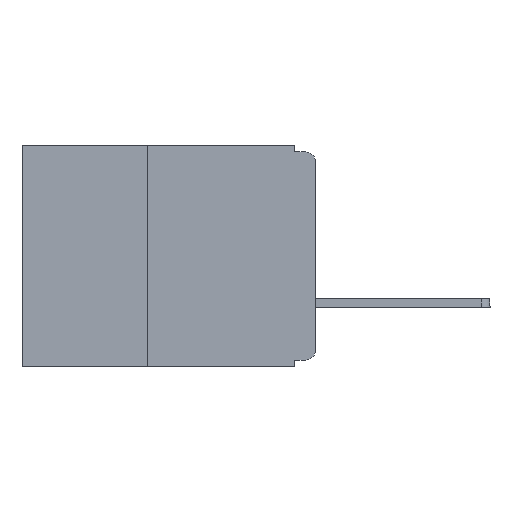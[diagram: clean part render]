
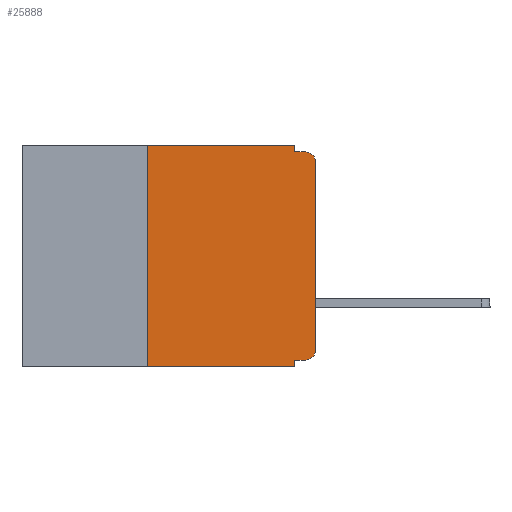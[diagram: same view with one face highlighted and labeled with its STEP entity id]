
A CAD part, left-side view. The second image highlights one B-rep face of the part: STEP entity #25888.
In plain terms, the highlighted planar face has unit normal (-1, 0, 0).
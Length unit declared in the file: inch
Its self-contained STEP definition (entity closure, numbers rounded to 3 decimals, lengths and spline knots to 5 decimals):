
#901 = AXIS2_PLACEMENT_3D ( 'NONE', #1587, #17180, #3846 ) ;
#1143 = CARTESIAN_POINT ( 'NONE',  ( 0., 0.015, -0.01 ) ) ;
#1209 = VECTOR ( 'NONE', #21143, 39.37008 ) ;
#1587 = CARTESIAN_POINT ( 'NONE',  ( 0., 0.015, -0.305 ) ) ;
#1785 = VERTEX_POINT ( 'NONE', #26968 ) ;
#2068 = VECTOR ( 'NONE', #14072, 39.37008 ) ;
#3245 = DIRECTION ( 'NONE',  ( 0., 0., 1. ) ) ;
#3846 = DIRECTION ( 'NONE',  ( 0., 0., -1. ) ) ;
#4267 = ORIENTED_EDGE ( 'NONE', *, *, #18179, .F. ) ;
#4443 = EDGE_CURVE ( 'NONE', #26422, #20674, #8044, .T. ) ;
#4678 = DIRECTION ( 'NONE',  ( 0., -1., 0. ) ) ;
#4700 = AXIS2_PLACEMENT_3D ( 'NONE', #23439, #10240, #25646 ) ;
#4774 = CARTESIAN_POINT ( 'NONE',  ( 0., 0.031, -0.01 ) ) ;
#4798 = CARTESIAN_POINT ( 'NONE',  ( 0., 0., -0.305 ) ) ;
#5119 = CARTESIAN_POINT ( 'NONE',  ( 0., 0.25, -0.33 ) ) ;
#5506 = EDGE_CURVE ( 'NONE', #12307, #23863, #15617, .T. ) ;
#5645 = CARTESIAN_POINT ( 'NONE',  ( 0., 0., -0.32 ) ) ;
#5861 = ORIENTED_EDGE ( 'NONE', *, *, #8614, .T. ) ;
#6112 = CARTESIAN_POINT ( 'NONE',  ( 0., 0.437, 0. ) ) ;
#6240 = VERTEX_POINT ( 'NONE', #17928 ) ;
#6316 = DIRECTION ( 'NONE',  ( 0., 0., -1. ) ) ;
#6658 = CARTESIAN_POINT ( 'NONE',  ( 0., 0.25, -0.33 ) ) ;
#6696 = AXIS2_PLACEMENT_3D ( 'NONE', #6112, #19563, #6316 ) ;
#7705 = CARTESIAN_POINT ( 'NONE',  ( 0., 0.031, -0.33 ) ) ;
#8044 = LINE ( 'NONE', #5119, #2068 ) ;
#8323 = VECTOR ( 'NONE', #3245, 39.37008 ) ;
#8610 = LINE ( 'NONE', #5645, #1209 ) ;
#8614 = EDGE_CURVE ( 'NONE', #26422, #23863, #14051, .T. ) ;
#8883 = CARTESIAN_POINT ( 'NONE',  ( 0., 0.031, -0.33 ) ) ;
#9052 = CIRCLE ( 'NONE', #901, 0.015 ) ;
#9238 = EDGE_CURVE ( 'NONE', #20674, #20779, #26025, .T. ) ;
#10240 = DIRECTION ( 'NONE',  ( -1., 0., 0. ) ) ;
#10681 = VERTEX_POINT ( 'NONE', #4798 ) ;
#10914 = ORIENTED_EDGE ( 'NONE', *, *, #5506, .F. ) ;
#11091 = DIRECTION ( 'NONE',  ( 0., 0., -1. ) ) ;
#11214 = VERTEX_POINT ( 'NONE', #4774 ) ;
#11258 = ORIENTED_EDGE ( 'NONE', *, *, #18445, .F. ) ;
#11495 = EDGE_LOOP ( 'NONE', ( #13450, #22256, #4267, #21321, #16335, #21779, #5861, #10914, #11258, #18236 ) ) ;
#11556 = EDGE_CURVE ( 'NONE', #1785, #10681, #9052, .T. ) ;
#12037 = EDGE_CURVE ( 'NONE', #10681, #6240, #25892, .T. ) ;
#12307 = VERTEX_POINT ( 'NONE', #12436 ) ;
#12436 = CARTESIAN_POINT ( 'NONE',  ( 0., 0.031, -0.32 ) ) ;
#12900 = CARTESIAN_POINT ( 'NONE',  ( 0., 0.437, -0.33 ) ) ;
#12923 = PLANE ( 'NONE',  #6696 ) ;
#12995 = DIRECTION ( 'NONE',  ( 0., -1., 0. ) ) ;
#13450 = ORIENTED_EDGE ( 'NONE', *, *, #12037, .T. ) ;
#13512 = CARTESIAN_POINT ( 'NONE',  ( 0., 0.25, 0. ) ) ;
#13808 = CARTESIAN_POINT ( 'NONE',  ( 0., 0.031, 0. ) ) ;
#14051 = LINE ( 'NONE', #12900, #25045 ) ;
#14072 = DIRECTION ( 'NONE',  ( 0., 0., 1. ) ) ;
#14208 = LINE ( 'NONE', #26830, #24513 ) ;
#14381 = CARTESIAN_POINT ( 'NONE',  ( 0., 0., 0. ) ) ;
#14649 = CIRCLE ( 'NONE', #4700, 0.015 ) ;
#14871 = LINE ( 'NONE', #17985, #15548 ) ;
#15548 = VECTOR ( 'NONE', #4678, 39.37008 ) ;
#15617 = LINE ( 'NONE', #8883, #26593 ) ;
#16335 = ORIENTED_EDGE ( 'NONE', *, *, #9238, .F. ) ;
#17180 = DIRECTION ( 'NONE',  ( -1., 0., 0. ) ) ;
#17778 = CARTESIAN_POINT ( 'NONE',  ( 0., 0.437, 0. ) ) ;
#17928 = CARTESIAN_POINT ( 'NONE',  ( 0., 0., -0.025 ) ) ;
#17985 = CARTESIAN_POINT ( 'NONE',  ( 0., 0., -0.01 ) ) ;
#18179 = EDGE_CURVE ( 'NONE', #11214, #23321, #14871, .T. ) ;
#18236 = ORIENTED_EDGE ( 'NONE', *, *, #11556, .T. ) ;
#18445 = EDGE_CURVE ( 'NONE', #1785, #12307, #8610, .T. ) ;
#19508 = VECTOR ( 'NONE', #19900, 39.37008 ) ;
#19563 = DIRECTION ( 'NONE',  ( 1., 0., 0. ) ) ;
#19900 = DIRECTION ( 'NONE',  ( 0., -1., 0. ) ) ;
#20423 = DIRECTION ( 'NONE',  ( 0., 0., -1. ) ) ;
#20674 = VERTEX_POINT ( 'NONE', #13512 ) ;
#20779 = VERTEX_POINT ( 'NONE', #13808 ) ;
#21143 = DIRECTION ( 'NONE',  ( 0., 1., 0. ) ) ;
#21321 = ORIENTED_EDGE ( 'NONE', *, *, #23143, .F. ) ;
#21641 = EDGE_CURVE ( 'NONE', #6240, #23321, #14649, .T. ) ;
#21779 = ORIENTED_EDGE ( 'NONE', *, *, #4443, .F. ) ;
#22256 = ORIENTED_EDGE ( 'NONE', *, *, #21641, .T. ) ;
#23143 = EDGE_CURVE ( 'NONE', #20779, #11214, #14208, .T. ) ;
#23321 = VERTEX_POINT ( 'NONE', #1143 ) ;
#23439 = CARTESIAN_POINT ( 'NONE',  ( 0., 0.015, -0.025 ) ) ;
#23863 = VERTEX_POINT ( 'NONE', #7705 ) ;
#24261 = FACE_OUTER_BOUND ( 'NONE', #11495, .T. ) ;
#24513 = VECTOR ( 'NONE', #20423, 39.37008 ) ;
#25045 = VECTOR ( 'NONE', #12995, 39.37008 ) ;
#25646 = DIRECTION ( 'NONE',  ( 0., 0., -1. ) ) ;
#25888 = ADVANCED_FACE ( 'NONE', ( #24261 ), #12923, .F. ) ;
#25892 = LINE ( 'NONE', #14381, #8323 ) ;
#26025 = LINE ( 'NONE', #17778, #19508 ) ;
#26422 = VERTEX_POINT ( 'NONE', #6658 ) ;
#26593 = VECTOR ( 'NONE', #11091, 39.37008 ) ;
#26830 = CARTESIAN_POINT ( 'NONE',  ( 0., 0.031, 0. ) ) ;
#26968 = CARTESIAN_POINT ( 'NONE',  ( 0., 0.015, -0.32 ) ) ;
